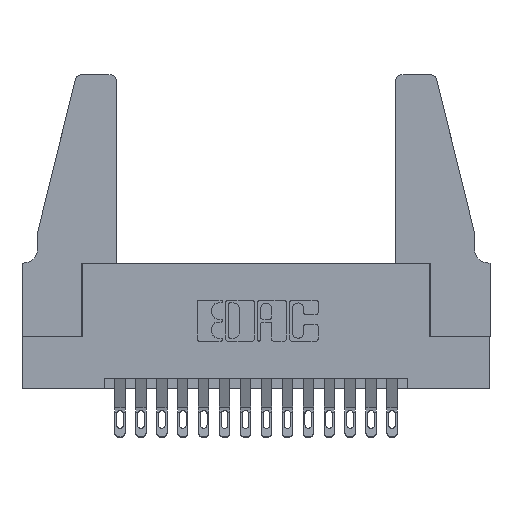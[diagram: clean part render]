
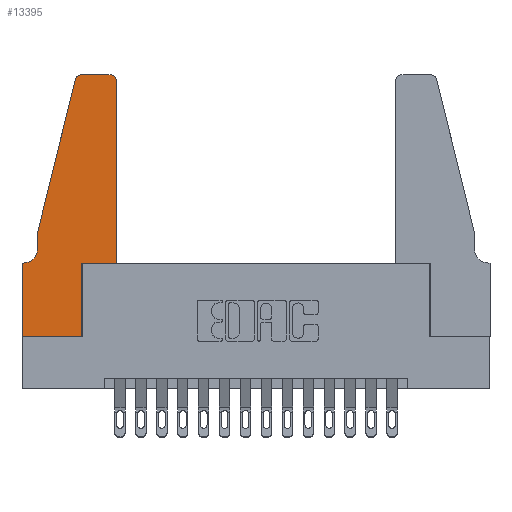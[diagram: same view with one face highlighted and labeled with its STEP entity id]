
A CAD part, top view. The second image highlights one B-rep face of the part: STEP entity #13395.
In plain terms, the highlighted planar face has unit normal (0, 0, 1).
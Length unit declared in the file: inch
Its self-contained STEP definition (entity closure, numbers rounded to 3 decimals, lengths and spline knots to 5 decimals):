
#206 = PLANE ( 'NONE',  #13023 ) ;
#414 = CARTESIAN_POINT ( 'NONE',  ( 0.2865, 0.35, 0.37 ) ) ;
#608 = CARTESIAN_POINT ( 'NONE',  ( 0.0755, 0.5, 0.37 ) ) ;
#1402 = VERTEX_POINT ( 'NONE', #10643 ) ;
#1486 = CIRCLE ( 'NONE', #12713, 0.07 ) ;
#1507 = FACE_OUTER_BOUND ( 'NONE', #14286, .T. ) ;
#1598 = DIRECTION ( 'NONE',  ( 1., 0., 0. ) ) ;
#1736 = VECTOR ( 'NONE', #7214, 39.37008 ) ;
#2026 = DIRECTION ( 'NONE',  ( -0.239, -0.971, 0. ) ) ;
#2174 = LINE ( 'NONE', #12440, #1736 ) ;
#2223 = VERTEX_POINT ( 'NONE', #4865 ) ;
#2295 = AXIS2_PLACEMENT_3D ( 'NONE', #11841, #3835, #13101 ) ;
#2597 = CARTESIAN_POINT ( 'NONE',  ( 0.0055, 0.42, 0.37 ) ) ;
#3059 = ORIENTED_EDGE ( 'NONE', *, *, #14250, .T. ) ;
#3390 = VERTEX_POINT ( 'NONE', #13574 ) ;
#3439 = CARTESIAN_POINT ( 'NONE',  ( 0.2865, 0.35, 0.37 ) ) ;
#3484 = LINE ( 'NONE', #15088, #3949 ) ;
#3594 = ORIENTED_EDGE ( 'NONE', *, *, #4815, .T. ) ;
#3640 = ORIENTED_EDGE ( 'NONE', *, *, #12772, .T. ) ;
#3679 = CARTESIAN_POINT ( 'NONE',  ( 0.4505, 0.35, 0.37 ) ) ;
#3725 = VECTOR ( 'NONE', #8796, 39.37008 ) ;
#3835 = DIRECTION ( 'NONE',  ( 0., 0., 1. ) ) ;
#3949 = VECTOR ( 'NONE', #9938, 39.37008 ) ;
#4003 = DIRECTION ( 'NONE',  ( -1., 0., 0. ) ) ;
#4093 = DIRECTION ( 'NONE',  ( 1., 0., 0. ) ) ;
#4172 = LINE ( 'NONE', #16530, #3725 ) ;
#4402 = DIRECTION ( 'NONE',  ( -1., 0., 0. ) ) ;
#4608 = AXIS2_PLACEMENT_3D ( 'NONE', #14314, #6509, #15634 ) ;
#4667 = CARTESIAN_POINT ( 'NONE',  ( 0.0755, 0.42, 0.37 ) ) ;
#4712 = EDGE_CURVE ( 'NONE', #7566, #11070, #2174, .T. ) ;
#4815 = EDGE_CURVE ( 'NONE', #2223, #7251, #4172, .T. ) ;
#4865 = CARTESIAN_POINT ( 'NONE',  ( 0.4505, 0.35, 0.37 ) ) ;
#5075 = ORIENTED_EDGE ( 'NONE', *, *, #16186, .T. ) ;
#5086 = DIRECTION ( 'NONE',  ( 1., 0., 0. ) ) ;
#5563 = ORIENTED_EDGE ( 'NONE', *, *, #13491, .T. ) ;
#6280 = CARTESIAN_POINT ( 'NONE',  ( 0.25487, 1.22718, 0.37 ) ) ;
#6327 = CARTESIAN_POINT ( 'NONE',  ( 0.2865, 0., 0.37 ) ) ;
#6509 = DIRECTION ( 'NONE',  ( 0., 0., 1. ) ) ;
#6826 = VECTOR ( 'NONE', #11273, 39.37008 ) ;
#7118 = CARTESIAN_POINT ( 'NONE',  ( 0.2605, 1.25, 0.37 ) ) ;
#7214 = DIRECTION ( 'NONE',  ( 0., -1., 0. ) ) ;
#7238 = LINE ( 'NONE', #414, #6826 ) ;
#7251 = VERTEX_POINT ( 'NONE', #17063 ) ;
#7566 = VERTEX_POINT ( 'NONE', #15099 ) ;
#8430 = DIRECTION ( 'NONE',  ( -1., 0., 0. ) ) ;
#8451 = CARTESIAN_POINT ( 'NONE',  ( 0., 0.35, 0.37 ) ) ;
#8796 = DIRECTION ( 'NONE',  ( 0., 1., 0. ) ) ;
#9024 = VERTEX_POINT ( 'NONE', #6327 ) ;
#9193 = ORIENTED_EDGE ( 'NONE', *, *, #15289, .T. ) ;
#9196 = LINE ( 'NONE', #3679, #15672 ) ;
#9728 = EDGE_CURVE ( 'NONE', #9024, #15751, #7238, .T. ) ;
#9769 = DIRECTION ( 'NONE',  ( 0., 0., 1. ) ) ;
#9938 = DIRECTION ( 'NONE',  ( 0., -1., 0. ) ) ;
#10074 = ORIENTED_EDGE ( 'NONE', *, *, #13849, .T. ) ;
#10154 = EDGE_CURVE ( 'NONE', #12715, #9024, #11797, .T. ) ;
#10373 = CARTESIAN_POINT ( 'NONE',  ( 0.284, 1.25, 0.37 ) ) ;
#10643 = CARTESIAN_POINT ( 'NONE',  ( 0.0055, 0.35, 0.37 ) ) ;
#10730 = ORIENTED_EDGE ( 'NONE', *, *, #11274, .T. ) ;
#11070 = VERTEX_POINT ( 'NONE', #4667 ) ;
#11093 = VECTOR ( 'NONE', #8430, 39.37008 ) ;
#11273 = DIRECTION ( 'NONE',  ( 0., 1., 0. ) ) ;
#11274 = EDGE_CURVE ( 'NONE', #7251, #3390, #11546, .T. ) ;
#11546 = CIRCLE ( 'NONE', #4608, 0.03 ) ;
#11563 = CARTESIAN_POINT ( 'NONE',  ( 0., 0.35, 0.37 ) ) ;
#11700 = VECTOR ( 'NONE', #4402, 39.37008 ) ;
#11720 = VERTEX_POINT ( 'NONE', #11563 ) ;
#11797 = LINE ( 'NONE', #17166, #14811 ) ;
#11822 = ORIENTED_EDGE ( 'NONE', *, *, #4712, .T. ) ;
#11841 = CARTESIAN_POINT ( 'NONE',  ( 0.284, 1.22, 0.37 ) ) ;
#11994 = DIRECTION ( 'NONE',  ( 0., 0., -1. ) ) ;
#12197 = ORIENTED_EDGE ( 'NONE', *, *, #10154, .T. ) ;
#12246 = CARTESIAN_POINT ( 'NONE',  ( 0., 0., 0.37 ) ) ;
#12361 = CARTESIAN_POINT ( 'NONE',  ( 0.0755, 0.35, 0.37 ) ) ;
#12440 = CARTESIAN_POINT ( 'NONE',  ( 0.0755, 0.5, 0.37 ) ) ;
#12713 = AXIS2_PLACEMENT_3D ( 'NONE', #2597, #11994, #4003 ) ;
#12715 = VERTEX_POINT ( 'NONE', #12246 ) ;
#12772 = EDGE_CURVE ( 'NONE', #3390, #16466, #14715, .T. ) ;
#13023 = AXIS2_PLACEMENT_3D ( 'NONE', #8451, #9769, #1598 ) ;
#13101 = DIRECTION ( 'NONE',  ( 1., 0., 0. ) ) ;
#13395 = ADVANCED_FACE ( 'NONE', ( #1507 ), #206, .T. ) ;
#13491 = EDGE_CURVE ( 'NONE', #11720, #12715, #3484, .T. ) ;
#13574 = CARTESIAN_POINT ( 'NONE',  ( 0.4205, 1.25, 0.37 ) ) ;
#13592 = EDGE_CURVE ( 'NONE', #14200, #7566, #16288, .T. ) ;
#13790 = ORIENTED_EDGE ( 'NONE', *, *, #9728, .T. ) ;
#13849 = EDGE_CURVE ( 'NONE', #11070, #1402, #1486, .T. ) ;
#14086 = LINE ( 'NONE', #12361, #11093 ) ;
#14200 = VERTEX_POINT ( 'NONE', #6280 ) ;
#14250 = EDGE_CURVE ( 'NONE', #15751, #2223, #9196, .T. ) ;
#14286 = EDGE_LOOP ( 'NONE', ( #3640, #9193, #17260, #11822, #10074, #5075, #5563, #12197, #13790, #3059, #3594, #10730 ) ) ;
#14314 = CARTESIAN_POINT ( 'NONE',  ( 0.4205, 1.22, 0.37 ) ) ;
#14715 = LINE ( 'NONE', #7118, #11700 ) ;
#14811 = VECTOR ( 'NONE', #4093, 39.37008 ) ;
#14951 = CIRCLE ( 'NONE', #2295, 0.03 ) ;
#15088 = CARTESIAN_POINT ( 'NONE',  ( 0., 0., 0.37 ) ) ;
#15099 = CARTESIAN_POINT ( 'NONE',  ( 0.0755, 0.5, 0.37 ) ) ;
#15289 = EDGE_CURVE ( 'NONE', #16466, #14200, #14951, .T. ) ;
#15634 = DIRECTION ( 'NONE',  ( 1., 0., 0. ) ) ;
#15672 = VECTOR ( 'NONE', #5086, 39.37008 ) ;
#15751 = VERTEX_POINT ( 'NONE', #3439 ) ;
#15899 = VECTOR ( 'NONE', #2026, 39.37008 ) ;
#16186 = EDGE_CURVE ( 'NONE', #1402, #11720, #14086, .T. ) ;
#16288 = LINE ( 'NONE', #608, #15899 ) ;
#16466 = VERTEX_POINT ( 'NONE', #10373 ) ;
#16530 = CARTESIAN_POINT ( 'NONE',  ( 0.4505, 0.35, 0.37 ) ) ;
#17063 = CARTESIAN_POINT ( 'NONE',  ( 0.4505, 1.22, 0.37 ) ) ;
#17166 = CARTESIAN_POINT ( 'NONE',  ( 0., 0., 0.37 ) ) ;
#17260 = ORIENTED_EDGE ( 'NONE', *, *, #13592, .T. ) ;
